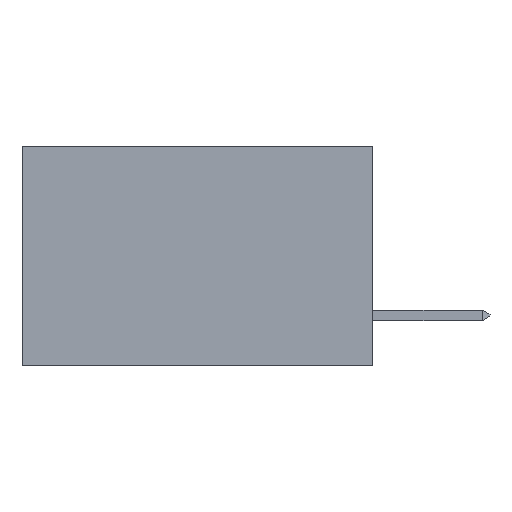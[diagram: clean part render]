
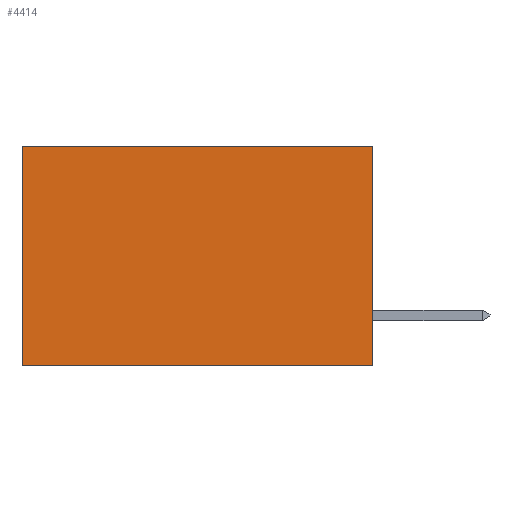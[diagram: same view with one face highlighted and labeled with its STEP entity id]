
A CAD part, left-side view. The second image highlights one B-rep face of the part: STEP entity #4414.
In plain terms, the highlighted planar face has unit normal (-1, 0, 0).
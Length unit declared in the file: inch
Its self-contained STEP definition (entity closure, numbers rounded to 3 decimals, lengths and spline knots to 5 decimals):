
#75 = EDGE_CURVE ( 'NONE', #662, #323, #908, .T. ) ;
#189 = VECTOR ( 'NONE', #8579, 39.37008 ) ;
#323 = VERTEX_POINT ( 'NONE', #5622 ) ;
#396 = VECTOR ( 'NONE', #7054, 39.37008 ) ;
#550 = AXIS2_PLACEMENT_3D ( 'NONE', #3056, #2659, #2579 ) ;
#662 = VERTEX_POINT ( 'NONE', #1618 ) ;
#908 = LINE ( 'NONE', #2942, #8354 ) ;
#1054 = EDGE_CURVE ( 'NONE', #323, #8095, #3914, .T. ) ;
#1618 = CARTESIAN_POINT ( 'NONE',  ( 0.277, 0., 0. ) ) ;
#1945 = VERTEX_POINT ( 'NONE', #7181 ) ;
#2198 = ORIENTED_EDGE ( 'NONE', *, *, #1054, .T. ) ;
#2219 = CARTESIAN_POINT ( 'NONE',  ( 0.277, 0.59, -0.37 ) ) ;
#2243 = LINE ( 'NONE', #8553, #189 ) ;
#2579 = DIRECTION ( 'NONE',  ( 0., 0., -1. ) ) ;
#2659 = DIRECTION ( 'NONE',  ( 1., 0., 0. ) ) ;
#2942 = CARTESIAN_POINT ( 'NONE',  ( 0.277, 0., 0. ) ) ;
#3045 = PLANE ( 'NONE',  #550 ) ;
#3056 = CARTESIAN_POINT ( 'NONE',  ( 0.277, 0., -0.37 ) ) ;
#3254 = VECTOR ( 'NONE', #8254, 39.37008 ) ;
#3914 = LINE ( 'NONE', #8470, #396 ) ;
#4414 = ADVANCED_FACE ( 'NONE', ( #8705 ), #3045, .F. ) ;
#4508 = EDGE_CURVE ( 'NONE', #1945, #8095, #2243, .T. ) ;
#4571 = EDGE_CURVE ( 'NONE', #662, #1945, #5796, .T. ) ;
#5081 = DIRECTION ( 'NONE',  ( 0., 1., 0. ) ) ;
#5133 = EDGE_LOOP ( 'NONE', ( #2198, #6375, #5728, #8202 ) ) ;
#5622 = CARTESIAN_POINT ( 'NONE',  ( 0.277, 0.59, 0. ) ) ;
#5728 = ORIENTED_EDGE ( 'NONE', *, *, #4571, .F. ) ;
#5796 = LINE ( 'NONE', #8167, #3254 ) ;
#6375 = ORIENTED_EDGE ( 'NONE', *, *, #4508, .F. ) ;
#7054 = DIRECTION ( 'NONE',  ( 0., 0., -1. ) ) ;
#7181 = CARTESIAN_POINT ( 'NONE',  ( 0.277, 0., -0.37 ) ) ;
#8095 = VERTEX_POINT ( 'NONE', #2219 ) ;
#8167 = CARTESIAN_POINT ( 'NONE',  ( 0.277, 0., -0.37 ) ) ;
#8202 = ORIENTED_EDGE ( 'NONE', *, *, #75, .T. ) ;
#8254 = DIRECTION ( 'NONE',  ( 0., 0., -1. ) ) ;
#8354 = VECTOR ( 'NONE', #5081, 39.37008 ) ;
#8470 = CARTESIAN_POINT ( 'NONE',  ( 0.277, 0.59, -0.37 ) ) ;
#8553 = CARTESIAN_POINT ( 'NONE',  ( 0.277, 0., -0.37 ) ) ;
#8579 = DIRECTION ( 'NONE',  ( 0., 1., 0. ) ) ;
#8705 = FACE_OUTER_BOUND ( 'NONE', #5133, .T. ) ;
